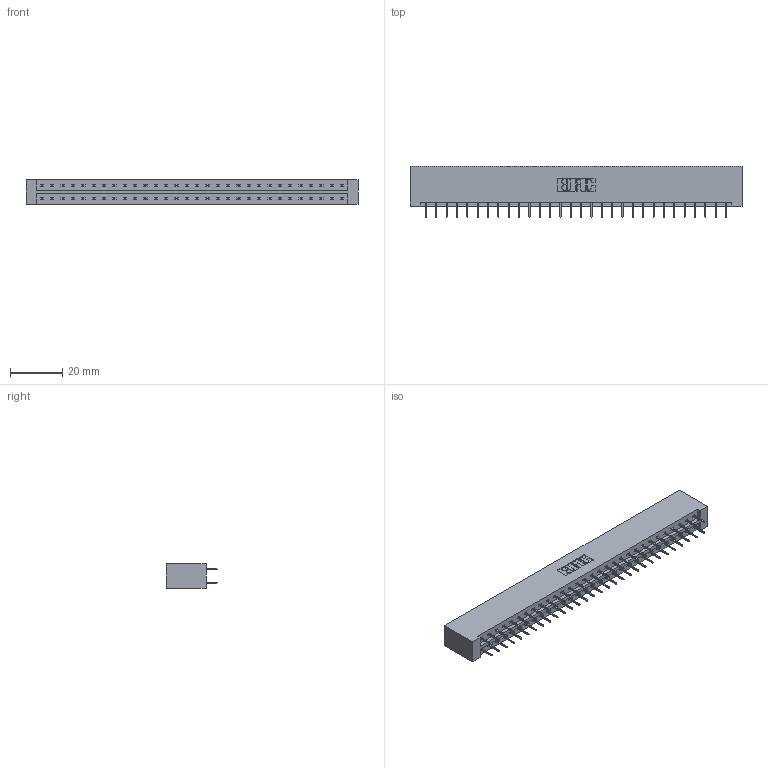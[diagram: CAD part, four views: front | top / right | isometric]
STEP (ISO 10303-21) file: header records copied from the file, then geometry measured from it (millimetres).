
FILE_DESCRIPTION (( 'STEP AP203' ), '1' );
FILE_NAME ('833-060-524-201.STEP', '2020-06-05T02:11:32', ( '' ), ( '' ), 'SwSTEP 2.0', 'SolidWorks 2020', '' );
FILE_SCHEMA (( 'CONFIG_CONTROL_DESIGN' ));
Length unit declared in the file: inch
Products named in the file (3): 833-060-524-201; 833 Part_Lugless; 345-292-001_345-293-124
Assembly tree (61 placements, depth 2):
  833-060-524-201
    833 Part_Lugless
    345-292-001_345-293-124  x60
Bounding box: 127.13 x 19.69 x 9.4 mm (x, y, z)
Volume: 13408.1 mm3; surface area: 15474.7 mm2
Topology: 61 solids, 61 shells, 3466 faces, 9827 edges, 6310 vertices
Faces by surface type: plane 2586, cylinder 880
Entity records: 20649 total; most frequent: CARTESIAN_POINT 3434, ORIENTED_EDGE 3370, DIRECTION 2949, EDGE_CURVE 1685, VECTOR 1569, LINE 1569, VERTEX_POINT 1118, AXIS2_PLACEMENT_3D 690
